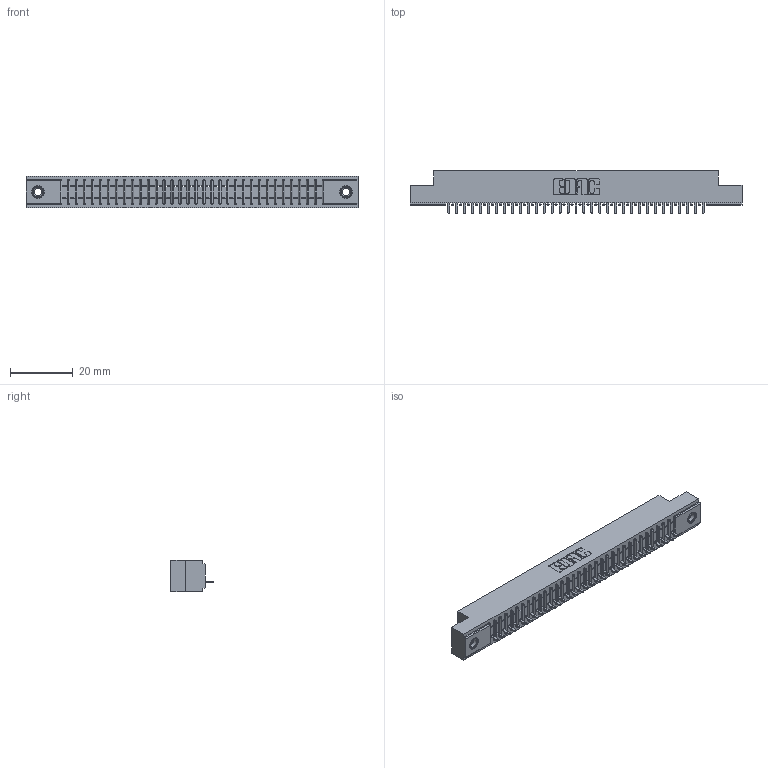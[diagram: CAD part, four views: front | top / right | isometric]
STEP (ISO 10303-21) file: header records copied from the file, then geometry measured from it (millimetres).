
FILE_DESCRIPTION (( 'STEP AP203' ), '1' );
FILE_NAME ('341-033-524-107.STEP', '2018-08-06T21:24:40', ( '' ), ( '' ), 'SwSTEP 2.0', 'SolidWorks 2016', '' );
FILE_SCHEMA (( 'CONFIG_CONTROL_DESIGN' ));
Length unit declared in the file: inch
Products named in the file (4): 341 Part_.156 (3.96) Dia Mounting Holes; 341-292-001_341-292-124; 345-250-001_345-250-005-103; 341-033-524-107
Assembly tree (36 placements, depth 2):
  341-033-524-107
    341 Part_.156 (3.96) Dia Mounting Holes
    341-292-001_341-292-124  x33
    345-250-001_345-250-005-103  x2
Bounding box: 106.05 x 13.64 x 10.16 mm (x, y, z)
Volume: 7570.2 mm3; surface area: 11482.2 mm2
Topology: 36 solids, 36 shells, 2882 faces, 8273 edges, 5306 vertices
Faces by surface type: plane 1783, cylinder 951, sphere 68, torus 68, cone 12
Entity records: 41265 total; most frequent: CARTESIAN_POINT 6985, ORIENTED_EDGE 6966, DIRECTION 6761, EDGE_CURVE 3483, VECTOR 2801, LINE 2801, VERTEX_POINT 2204, AXIS2_PLACEMENT_3D 1980
